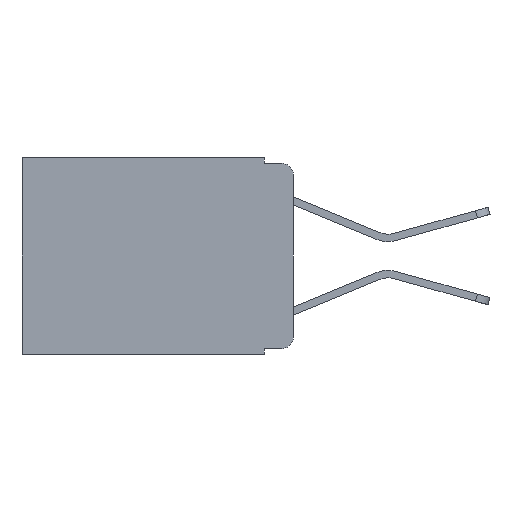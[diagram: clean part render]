
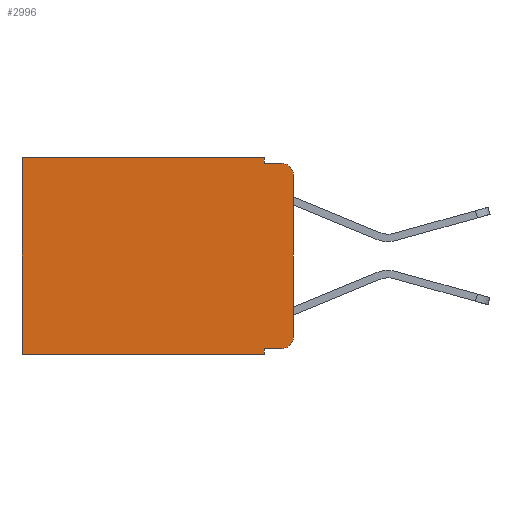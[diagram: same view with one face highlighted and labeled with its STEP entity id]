
A CAD part, left-side view. The second image highlights one B-rep face of the part: STEP entity #2996.
In plain terms, the highlighted planar face has unit normal (-1, 0, 0).
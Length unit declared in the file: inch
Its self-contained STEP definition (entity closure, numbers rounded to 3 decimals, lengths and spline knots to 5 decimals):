
#45 = LINE ( 'NONE', #13356, #3516 ) ;
#416 = LINE ( 'NONE', #11219, #7404 ) ;
#464 = LINE ( 'NONE', #4589, #10036 ) ;
#519 = EDGE_CURVE ( 'NONE', #10352, #8238, #464, .T. ) ;
#618 = VECTOR ( 'NONE', #15922, 39.37008 ) ;
#739 = AXIS2_PLACEMENT_3D ( 'NONE', #2793, #2713, #5536 ) ;
#1024 = CARTESIAN_POINT ( 'NONE',  ( 0.298, 0., 0. ) ) ;
#1190 = PLANE ( 'NONE',  #16378 ) ;
#1343 = EDGE_CURVE ( 'NONE', #12756, #8238, #416, .T. ) ;
#1617 = EDGE_CURVE ( 'NONE', #10636, #12756, #12812, .T. ) ;
#1760 = DIRECTION ( 'NONE',  ( 0., -1., 0. ) ) ;
#1840 = DIRECTION ( 'NONE',  ( 0., 0., -1. ) ) ;
#1966 = DIRECTION ( 'NONE',  ( 1., 0., 0. ) ) ;
#2544 = EDGE_CURVE ( 'NONE', #10636, #4092, #13207, .T. ) ;
#2548 = VERTEX_POINT ( 'NONE', #13331 ) ;
#2678 = DIRECTION ( 'NONE',  ( 0., 1., 0. ) ) ;
#2713 = DIRECTION ( 'NONE',  ( -1., 0., 0. ) ) ;
#2723 = CARTESIAN_POINT ( 'NONE',  ( 0.298, 0.473, -0.343 ) ) ;
#2793 = CARTESIAN_POINT ( 'NONE',  ( 0.298, 0.02, -0.313 ) ) ;
#2996 = ADVANCED_FACE ( 'NONE', ( #13380 ), #1190, .F. ) ;
#3023 = DIRECTION ( 'NONE',  ( 0., 0., -1. ) ) ;
#3216 = DIRECTION ( 'NONE',  ( 0., 0., -1. ) ) ;
#3435 = EDGE_CURVE ( 'NONE', #4092, #8425, #5840, .T. ) ;
#3516 = VECTOR ( 'NONE', #1760, 39.37008 ) ;
#3739 = CARTESIAN_POINT ( 'NONE',  ( 0.298, 0.473, 0. ) ) ;
#4092 = VERTEX_POINT ( 'NONE', #4493 ) ;
#4490 = VECTOR ( 'NONE', #15034, 39.37008 ) ;
#4493 = CARTESIAN_POINT ( 'NONE',  ( 0.298, 0.02, -0.333 ) ) ;
#4570 = DIRECTION ( 'NONE',  ( 0., 0., -1. ) ) ;
#4589 = CARTESIAN_POINT ( 'NONE',  ( 0.298, 0.473, 0. ) ) ;
#4630 = CARTESIAN_POINT ( 'NONE',  ( 0.298, 0.051, 0. ) ) ;
#4799 = ORIENTED_EDGE ( 'NONE', *, *, #14866, .F. ) ;
#4845 = ORIENTED_EDGE ( 'NONE', *, *, #10794, .F. ) ;
#5066 = CIRCLE ( 'NONE', #5225, 0.02 ) ;
#5148 = DIRECTION ( 'NONE',  ( -1., 0., 0. ) ) ;
#5225 = AXIS2_PLACEMENT_3D ( 'NONE', #12730, #5148, #13993 ) ;
#5536 = DIRECTION ( 'NONE',  ( 0., 0., -1. ) ) ;
#5840 = CIRCLE ( 'NONE', #739, 0.02 ) ;
#6664 = VECTOR ( 'NONE', #3216, 39.37008 ) ;
#6832 = CARTESIAN_POINT ( 'NONE',  ( 0.298, 0., -0.03 ) ) ;
#7404 = VECTOR ( 'NONE', #2678, 39.37008 ) ;
#7856 = CARTESIAN_POINT ( 'NONE',  ( 0.298, 0.051, -0.343 ) ) ;
#8238 = VERTEX_POINT ( 'NONE', #2723 ) ;
#8425 = VERTEX_POINT ( 'NONE', #12166 ) ;
#8651 = CARTESIAN_POINT ( 'NONE',  ( 0.298, 0.051, 0. ) ) ;
#8653 = CARTESIAN_POINT ( 'NONE',  ( 0.298, 0., 0. ) ) ;
#9537 = EDGE_CURVE ( 'NONE', #12380, #10352, #11326, .T. ) ;
#9586 = VECTOR ( 'NONE', #3023, 39.37008 ) ;
#9797 = VERTEX_POINT ( 'NONE', #11988 ) ;
#9811 = ORIENTED_EDGE ( 'NONE', *, *, #3435, .T. ) ;
#9974 = VECTOR ( 'NONE', #13277, 39.37008 ) ;
#10036 = VECTOR ( 'NONE', #4570, 39.37008 ) ;
#10352 = VERTEX_POINT ( 'NONE', #3739 ) ;
#10636 = VERTEX_POINT ( 'NONE', #11921 ) ;
#10794 = EDGE_CURVE ( 'NONE', #14655, #8425, #11293, .T. ) ;
#11219 = CARTESIAN_POINT ( 'NONE',  ( 0.298, 0., -0.343 ) ) ;
#11242 = ORIENTED_EDGE ( 'NONE', *, *, #15637, .F. ) ;
#11293 = LINE ( 'NONE', #8653, #618 ) ;
#11326 = LINE ( 'NONE', #12570, #4490 ) ;
#11921 = CARTESIAN_POINT ( 'NONE',  ( 0.298, 0.051, -0.333 ) ) ;
#11988 = CARTESIAN_POINT ( 'NONE',  ( 0.298, 0.02, -0.01 ) ) ;
#12002 = ORIENTED_EDGE ( 'NONE', *, *, #1343, .F. ) ;
#12166 = CARTESIAN_POINT ( 'NONE',  ( 0.298, 0., -0.313 ) ) ;
#12223 = CARTESIAN_POINT ( 'NONE',  ( 0.298, 0.051, -0.333 ) ) ;
#12380 = VERTEX_POINT ( 'NONE', #16809 ) ;
#12570 = CARTESIAN_POINT ( 'NONE',  ( 0.298, 0., 0. ) ) ;
#12730 = CARTESIAN_POINT ( 'NONE',  ( 0.298, 0.02, -0.03 ) ) ;
#12756 = VERTEX_POINT ( 'NONE', #7856 ) ;
#12812 = LINE ( 'NONE', #8651, #9586 ) ;
#13050 = ORIENTED_EDGE ( 'NONE', *, *, #2544, .T. ) ;
#13183 = ORIENTED_EDGE ( 'NONE', *, *, #9537, .T. ) ;
#13207 = LINE ( 'NONE', #12223, #9974 ) ;
#13235 = EDGE_CURVE ( 'NONE', #14655, #9797, #5066, .T. ) ;
#13277 = DIRECTION ( 'NONE',  ( 0., -1., 0. ) ) ;
#13331 = CARTESIAN_POINT ( 'NONE',  ( 0.298, 0.051, -0.01 ) ) ;
#13356 = CARTESIAN_POINT ( 'NONE',  ( 0.298, 0.051, -0.01 ) ) ;
#13380 = FACE_OUTER_BOUND ( 'NONE', #15724, .T. ) ;
#13619 = ORIENTED_EDGE ( 'NONE', *, *, #519, .T. ) ;
#13993 = DIRECTION ( 'NONE',  ( 0., 0., -1. ) ) ;
#14655 = VERTEX_POINT ( 'NONE', #6832 ) ;
#14866 = EDGE_CURVE ( 'NONE', #2548, #9797, #45, .T. ) ;
#15034 = DIRECTION ( 'NONE',  ( 0., 1., 0. ) ) ;
#15637 = EDGE_CURVE ( 'NONE', #12380, #2548, #16512, .T. ) ;
#15724 = EDGE_LOOP ( 'NONE', ( #4845, #16320, #4799, #11242, #13183, #13619, #12002, #16611, #13050, #9811 ) ) ;
#15922 = DIRECTION ( 'NONE',  ( 0., 0., -1. ) ) ;
#16320 = ORIENTED_EDGE ( 'NONE', *, *, #13235, .T. ) ;
#16378 = AXIS2_PLACEMENT_3D ( 'NONE', #1024, #1966, #1840 ) ;
#16512 = LINE ( 'NONE', #4630, #6664 ) ;
#16611 = ORIENTED_EDGE ( 'NONE', *, *, #1617, .F. ) ;
#16809 = CARTESIAN_POINT ( 'NONE',  ( 0.298, 0.051, 0. ) ) ;
